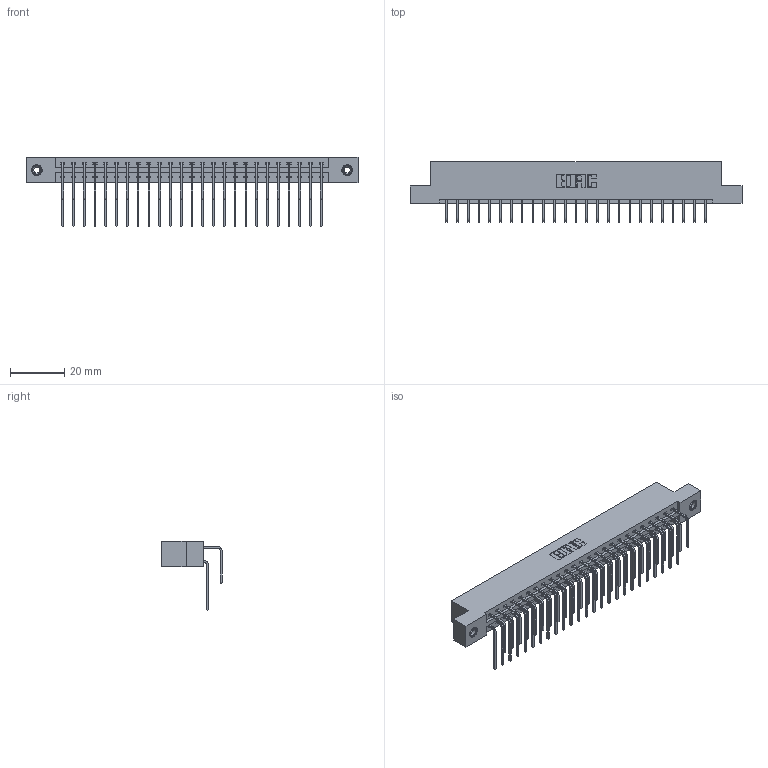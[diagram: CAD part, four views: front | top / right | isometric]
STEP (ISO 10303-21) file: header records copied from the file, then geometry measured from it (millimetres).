
FILE_DESCRIPTION (( 'STEP AP203' ), '1' );
FILE_NAME ('387-050-558-208.STEP', '2018-09-20T09:04:52', ( '' ), ( '' ), 'SwSTEP 2.0', 'SolidWorks 2016', '' );
FILE_SCHEMA (( 'CONFIG_CONTROL_DESIGN' ));
Length unit declared in the file: inch
Products named in the file (5): 337 Part_Flush Mounting Lugs - 0.156 Dia-TI; 345-292-001_558 559 Tail - 1; 345-292-001_558 Tail - 2; 345-250-001_345-250-003-102; 387-050-558-208
Assembly tree (53 placements, depth 2):
  387-050-558-208
    337 Part_Flush Mounting Lugs - 0.156 Dia-TI
    345-292-001_558 559 Tail - 1  x25
    345-292-001_558 Tail - 2  x25
    345-250-001_345-250-003-102  x2
Bounding box: 122.07 x 22.17 x 25.53 mm (x, y, z)
Volume: 12920.6 mm3; surface area: 15913.9 mm2
Topology: 53 solids, 53 shells, 2974 faces, 8797 edges, 5790 vertices
Faces by surface type: plane 2102, cylinder 856, cone 12, torus 4
Entity records: 24552 total; most frequent: CARTESIAN_POINT 4176, ORIENTED_EDGE 4054, DIRECTION 3597, EDGE_CURVE 2027, LINE 1839, VECTOR 1839, VERTEX_POINT 1344, AXIS2_PLACEMENT_3D 879
